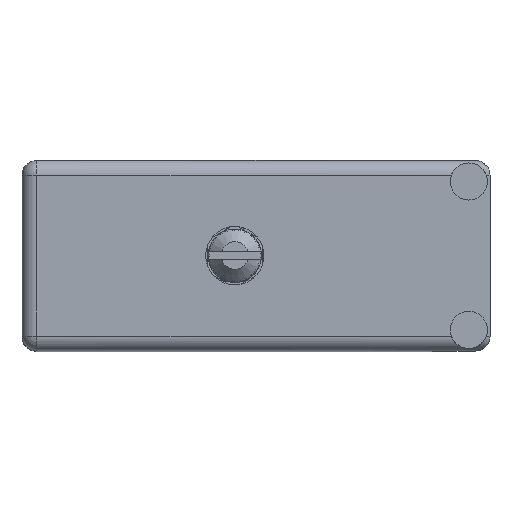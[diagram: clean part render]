
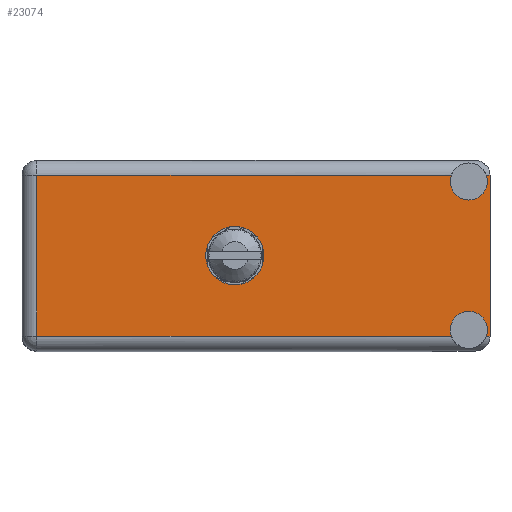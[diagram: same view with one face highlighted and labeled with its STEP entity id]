
A CAD part, top view. The second image highlights one B-rep face of the part: STEP entity #23074.
In plain terms, the highlighted face is planar.
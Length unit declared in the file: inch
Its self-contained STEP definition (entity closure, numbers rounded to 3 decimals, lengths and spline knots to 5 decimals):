
#270 = ORIENTED_EDGE ( 'NONE', *, *, #1631, .F. ) ;
#1631 = EDGE_CURVE ( 'NONE', #59051, #61739, #9384, .T. ) ;
#2054 = EDGE_CURVE ( 'NONE', #111758, #25639, #51293, .T. ) ;
#2415 = CARTESIAN_POINT ( 'NONE',  ( -1.004, 1.466, -0.4495 ) ) ;
#4591 = ORIENTED_EDGE ( 'NONE', *, *, #2054, .T. ) ;
#5137 = ORIENTED_EDGE ( 'NONE', *, *, #42974, .T. ) ;
#5585 = AXIS2_PLACEMENT_3D ( 'NONE', #14682, #50103, #109337 ) ;
#5787 = VERTEX_POINT ( 'NONE', #85011 ) ;
#6216 = CIRCLE ( 'NONE', #28482, 0.0875 ) ;
#7661 = CARTESIAN_POINT ( 'NONE',  ( -0.934, 1.466, 0.3795 ) ) ;
#8186 = DIRECTION ( 'NONE',  ( 0., 0., 1. ) ) ;
#9306 = AXIS2_PLACEMENT_3D ( 'NONE', #73946, #91958, #55971 ) ;
#9384 = CIRCLE ( 'NONE', #9306, 0.1375 ) ;
#9961 = PLANE ( 'NONE',  #84474 ) ;
#11303 = VECTOR ( 'NONE', #66993, 39.37008 ) ;
#12515 = EDGE_CURVE ( 'NONE', #5787, #66710, #84354, .T. ) ;
#12749 = DIRECTION ( 'NONE',  ( 0., 0., 1. ) ) ;
#12794 = CARTESIAN_POINT ( 'NONE',  ( 0., 1.466, 0. ) ) ;
#13171 = VECTOR ( 'NONE', #80992, 39.37008 ) ;
#13315 = DIRECTION ( 'NONE',  ( 0., 1., 0. ) ) ;
#13933 = DIRECTION ( 'NONE',  ( 0., 1., 0. ) ) ;
#14626 = CARTESIAN_POINT ( 'NONE',  ( -1.004, 1.466, -0.3795 ) ) ;
#14682 = CARTESIAN_POINT ( 'NONE',  ( 1.104, 1.466, -0.35 ) ) ;
#14749 = CARTESIAN_POINT ( 'NONE',  ( 1.204, 1.466, 0.3795 ) ) ;
#15161 = VERTEX_POINT ( 'NONE', #98101 ) ;
#16944 = ORIENTED_EDGE ( 'NONE', *, *, #39389, .F. ) ;
#18323 = CARTESIAN_POINT ( 'NONE',  ( 1.104, 1.466, 0.2625 ) ) ;
#19246 = DIRECTION ( 'NONE',  ( -1., 0., 0. ) ) ;
#19470 = CARTESIAN_POINT ( 'NONE',  ( -1.004, 1.466, -0.3795 ) ) ;
#19542 = EDGE_CURVE ( 'NONE', #22802, #66205, #88638, .T. ) ;
#22802 = VERTEX_POINT ( 'NONE', #68076 ) ;
#23074 = ADVANCED_FACE ( 'NONE', ( #81908, #98188 ), #9961, .T. ) ;
#25639 = VERTEX_POINT ( 'NONE', #45533 ) ;
#27538 = DIRECTION ( 'NONE',  ( 0., 1., 0. ) ) ;
#27663 = EDGE_LOOP ( 'NONE', ( #4591, #58826, #94249, #28587, #16944, #5137, #94600, #52193, #69818, #85453 ) ) ;
#28482 = AXIS2_PLACEMENT_3D ( 'NONE', #107654, #27538, #62942 ) ;
#28587 = ORIENTED_EDGE ( 'NONE', *, *, #19542, .T. ) ;
#28673 = VECTOR ( 'NONE', #53777, 39.37008 ) ;
#35574 = ORIENTED_EDGE ( 'NONE', *, *, #44357, .F. ) ;
#37593 = EDGE_LOOP ( 'NONE', ( #35574, #270 ) ) ;
#37775 = DIRECTION ( 'NONE',  ( 0., 1., 0. ) ) ;
#39389 = EDGE_CURVE ( 'NONE', #15161, #66205, #107608, .T. ) ;
#39514 = EDGE_CURVE ( 'NONE', #66710, #43119, #42591, .T. ) ;
#40789 = CARTESIAN_POINT ( 'NONE',  ( -0.934, 1.466, -0.3795 ) ) ;
#41867 = DIRECTION ( 'NONE',  ( 0., 1., 0. ) ) ;
#42591 = CIRCLE ( 'NONE', #5585, 0.0875 ) ;
#42974 = EDGE_CURVE ( 'NONE', #15161, #43119, #107153, .T. ) ;
#43119 = VERTEX_POINT ( 'NONE', #111178 ) ;
#44357 = EDGE_CURVE ( 'NONE', #61739, #59051, #113553, .T. ) ;
#44914 = DIRECTION ( 'NONE',  ( 0., 0., 1. ) ) ;
#45533 = CARTESIAN_POINT ( 'NONE',  ( 1.02162, 1.466, 0.3795 ) ) ;
#47835 = EDGE_CURVE ( 'NONE', #91100, #25639, #6216, .T. ) ;
#49124 = AXIS2_PLACEMENT_3D ( 'NONE', #87725, #41867, #8186 ) ;
#49150 = AXIS2_PLACEMENT_3D ( 'NONE', #108543, #13315, #12749 ) ;
#50103 = DIRECTION ( 'NONE',  ( 0., 1., 0. ) ) ;
#51293 = LINE ( 'NONE', #14749, #11303 ) ;
#52193 = ORIENTED_EDGE ( 'NONE', *, *, #12515, .F. ) ;
#53777 = DIRECTION ( 'NONE',  ( 1., 0., 0. ) ) ;
#55197 = EDGE_CURVE ( 'NONE', #5787, #99451, #94155, .T. ) ;
#55971 = DIRECTION ( 'NONE',  ( 0., 0., 1. ) ) ;
#57731 = VECTOR ( 'NONE', #104844, 39.37008 ) ;
#58060 = DIRECTION ( 'NONE',  ( 0., 0., 1. ) ) ;
#58826 = ORIENTED_EDGE ( 'NONE', *, *, #47835, .F. ) ;
#59051 = VERTEX_POINT ( 'NONE', #86596 ) ;
#61739 = VERTEX_POINT ( 'NONE', #91055 ) ;
#62104 = CIRCLE ( 'NONE', #49124, 0.0875 ) ;
#62942 = DIRECTION ( 'NONE',  ( 0., 0., 1. ) ) ;
#63459 = AXIS2_PLACEMENT_3D ( 'NONE', #12794, #13933, #58060 ) ;
#66205 = VERTEX_POINT ( 'NONE', #108981 ) ;
#66710 = VERTEX_POINT ( 'NONE', #78568 ) ;
#66993 = DIRECTION ( 'NONE',  ( 1., 0., 0. ) ) ;
#68076 = CARTESIAN_POINT ( 'NONE',  ( 1.18638, 1.466, 0.3795 ) ) ;
#69818 = ORIENTED_EDGE ( 'NONE', *, *, #55197, .T. ) ;
#73946 = CARTESIAN_POINT ( 'NONE',  ( 0., 1.466, 0. ) ) ;
#78568 = CARTESIAN_POINT ( 'NONE',  ( 1.104, 1.466, -0.2625 ) ) ;
#79693 = VECTOR ( 'NONE', #94732, 39.37008 ) ;
#80992 = DIRECTION ( 'NONE',  ( -1., 0., 0. ) ) ;
#81020 = CARTESIAN_POINT ( 'NONE',  ( 1.204, 1.466, 0.3795 ) ) ;
#81460 = CARTESIAN_POINT ( 'NONE',  ( 1.204, 1.466, 0.4495 ) ) ;
#81908 = FACE_BOUND ( 'NONE', #37593, .T. ) ;
#82135 = EDGE_CURVE ( 'NONE', #99451, #111758, #105427, .T. ) ;
#84354 = CIRCLE ( 'NONE', #49150, 0.0875 ) ;
#84474 = AXIS2_PLACEMENT_3D ( 'NONE', #2415, #37775, #19246 ) ;
#85011 = CARTESIAN_POINT ( 'NONE',  ( 1.02162, 1.466, -0.3795 ) ) ;
#85453 = ORIENTED_EDGE ( 'NONE', *, *, #82135, .T. ) ;
#86596 = CARTESIAN_POINT ( 'NONE',  ( 0., 1.466, -0.1375 ) ) ;
#87725 = CARTESIAN_POINT ( 'NONE',  ( 1.104, 1.466, 0.35 ) ) ;
#88638 = LINE ( 'NONE', #81020, #28673 ) ;
#91055 = CARTESIAN_POINT ( 'NONE',  ( 0., 1.466, 0.1375 ) ) ;
#91100 = VERTEX_POINT ( 'NONE', #18323 ) ;
#91958 = DIRECTION ( 'NONE',  ( 0., 1., 0. ) ) ;
#94155 = LINE ( 'NONE', #14626, #79693 ) ;
#94249 = ORIENTED_EDGE ( 'NONE', *, *, #110375, .F. ) ;
#94600 = ORIENTED_EDGE ( 'NONE', *, *, #39514, .F. ) ;
#94732 = DIRECTION ( 'NONE',  ( -1., 0., 0. ) ) ;
#98101 = CARTESIAN_POINT ( 'NONE',  ( 1.204, 1.466, -0.3795 ) ) ;
#98188 = FACE_OUTER_BOUND ( 'NONE', #27663, .T. ) ;
#99451 = VERTEX_POINT ( 'NONE', #40789 ) ;
#103695 = CARTESIAN_POINT ( 'NONE',  ( -0.934, 1.466, -0.4495 ) ) ;
#104844 = DIRECTION ( 'NONE',  ( 0., 0., 1. ) ) ;
#105427 = LINE ( 'NONE', #103695, #57731 ) ;
#107153 = LINE ( 'NONE', #19470, #13171 ) ;
#107489 = VECTOR ( 'NONE', #44914, 39.37008 ) ;
#107608 = LINE ( 'NONE', #81460, #107489 ) ;
#107654 = CARTESIAN_POINT ( 'NONE',  ( 1.104, 1.466, 0.35 ) ) ;
#108543 = CARTESIAN_POINT ( 'NONE',  ( 1.104, 1.466, -0.35 ) ) ;
#108981 = CARTESIAN_POINT ( 'NONE',  ( 1.204, 1.466, 0.3795 ) ) ;
#109337 = DIRECTION ( 'NONE',  ( 0., 0., 1. ) ) ;
#110375 = EDGE_CURVE ( 'NONE', #22802, #91100, #62104, .T. ) ;
#111178 = CARTESIAN_POINT ( 'NONE',  ( 1.18638, 1.466, -0.3795 ) ) ;
#111758 = VERTEX_POINT ( 'NONE', #7661 ) ;
#113553 = CIRCLE ( 'NONE', #63459, 0.1375 ) ;
